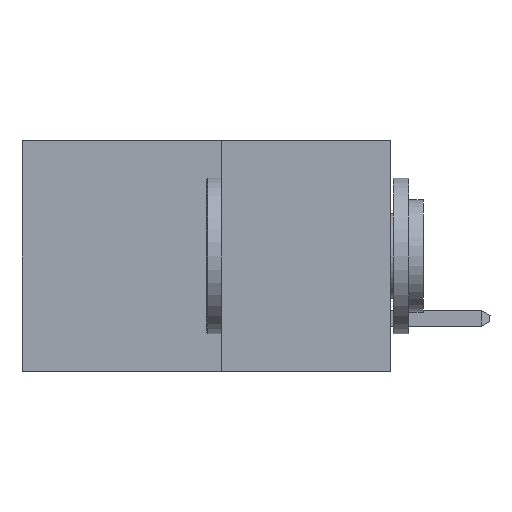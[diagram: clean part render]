
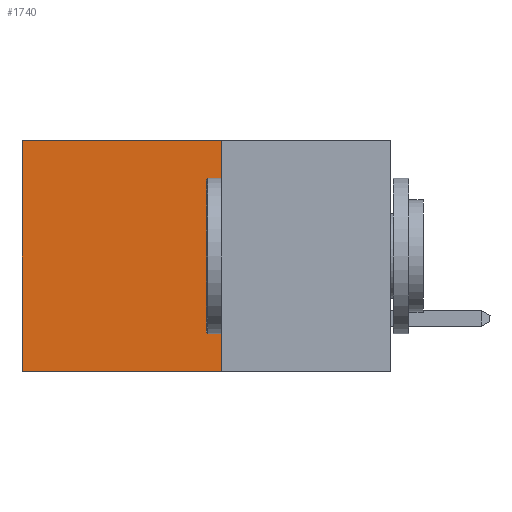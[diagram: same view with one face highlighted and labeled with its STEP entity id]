
A CAD part, left-side view. The second image highlights one B-rep face of the part: STEP entity #1740.
In plain terms, the highlighted planar face has unit normal (-1, 0, 0).
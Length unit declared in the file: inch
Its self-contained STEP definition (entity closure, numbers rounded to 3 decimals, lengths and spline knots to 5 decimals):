
#33 = VERTEX_POINT ( 'NONE', #7856 ) ;
#345 = DIRECTION ( 'NONE',  ( 0., 1., 0. ) ) ;
#1263 = ORIENTED_EDGE ( 'NONE', *, *, #8429, .T. ) ;
#1411 = ORIENTED_EDGE ( 'NONE', *, *, #3319, .F. ) ;
#1432 = VERTEX_POINT ( 'NONE', #2914 ) ;
#1654 = DIRECTION ( 'NONE',  ( 0., 0., -1. ) ) ;
#1725 = VERTEX_POINT ( 'NONE', #2201 ) ;
#1740 = ADVANCED_FACE ( 'NONE', ( #9345 ), #2251, .F. ) ;
#1854 = VECTOR ( 'NONE', #9886, 39.37008 ) ;
#2053 = ORIENTED_EDGE ( 'NONE', *, *, #4198, .F. ) ;
#2195 = CARTESIAN_POINT ( 'NONE',  ( 0.277, 0.59, -0.37 ) ) ;
#2201 = CARTESIAN_POINT ( 'NONE',  ( 0.277, 0.59, -0.37 ) ) ;
#2251 = PLANE ( 'NONE',  #4024 ) ;
#2318 = VECTOR ( 'NONE', #3242, 39.37008 ) ;
#2446 = LINE ( 'NONE', #2556, #6594 ) ;
#2556 = CARTESIAN_POINT ( 'NONE',  ( 0.277, 0.27, -0.37 ) ) ;
#2585 = ORIENTED_EDGE ( 'NONE', *, *, #4050, .T. ) ;
#2914 = CARTESIAN_POINT ( 'NONE',  ( 0.277, 0.27, -0.37 ) ) ;
#3242 = DIRECTION ( 'NONE',  ( 0., 0., -1. ) ) ;
#3319 = EDGE_CURVE ( 'NONE', #1432, #1725, #2446, .T. ) ;
#4024 = AXIS2_PLACEMENT_3D ( 'NONE', #9841, #9820, #1654 ) ;
#4050 = EDGE_CURVE ( 'NONE', #8226, #33, #5864, .T. ) ;
#4198 = EDGE_CURVE ( 'NONE', #8226, #1432, #4729, .T. ) ;
#4316 = CARTESIAN_POINT ( 'NONE',  ( 0.277, 0.27, -0.37 ) ) ;
#4729 = LINE ( 'NONE', #4316, #2318 ) ;
#5162 = CARTESIAN_POINT ( 'NONE',  ( 0.277, 0.27, 0. ) ) ;
#5716 = CARTESIAN_POINT ( 'NONE',  ( 0.277, 0.27, 0. ) ) ;
#5864 = LINE ( 'NONE', #5716, #6121 ) ;
#6006 = DIRECTION ( 'NONE',  ( 0., 1., 0. ) ) ;
#6121 = VECTOR ( 'NONE', #6006, 39.37008 ) ;
#6594 = VECTOR ( 'NONE', #345, 39.37008 ) ;
#7856 = CARTESIAN_POINT ( 'NONE',  ( 0.277, 0.59, 0. ) ) ;
#8226 = VERTEX_POINT ( 'NONE', #5162 ) ;
#8429 = EDGE_CURVE ( 'NONE', #33, #1725, #9816, .T. ) ;
#9345 = FACE_OUTER_BOUND ( 'NONE', #10003, .T. ) ;
#9816 = LINE ( 'NONE', #2195, #1854 ) ;
#9820 = DIRECTION ( 'NONE',  ( 1., 0., 0. ) ) ;
#9841 = CARTESIAN_POINT ( 'NONE',  ( 0.277, 0.27, -0.37 ) ) ;
#9886 = DIRECTION ( 'NONE',  ( 0., 0., -1. ) ) ;
#10003 = EDGE_LOOP ( 'NONE', ( #1263, #1411, #2053, #2585 ) ) ;
